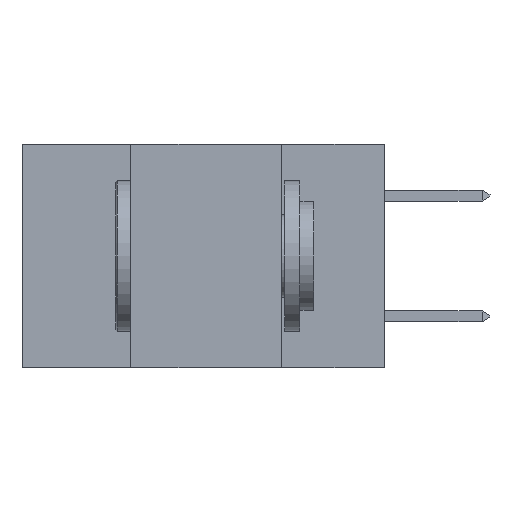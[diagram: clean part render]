
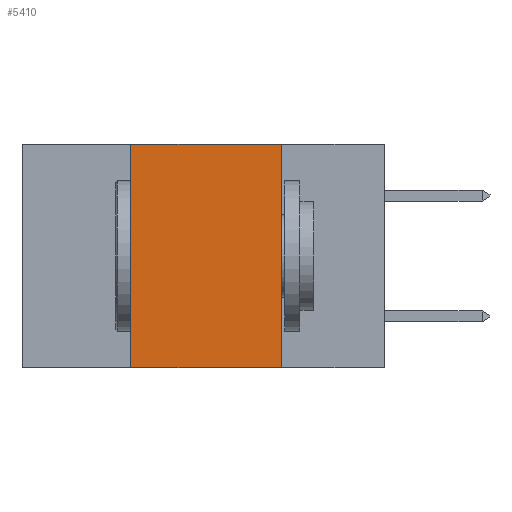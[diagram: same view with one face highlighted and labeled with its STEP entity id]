
A CAD part, left-side view. The second image highlights one B-rep face of the part: STEP entity #5410.
In plain terms, the highlighted planar face has unit normal (-1, 0, 0).
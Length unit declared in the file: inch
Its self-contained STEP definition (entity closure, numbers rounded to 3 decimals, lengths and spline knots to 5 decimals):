
#563 = VECTOR ( 'NONE', #12512, 39.37008 ) ;
#585 = LINE ( 'NONE', #1624, #803 ) ;
#803 = VECTOR ( 'NONE', #5555, 39.37008 ) ;
#886 = ORIENTED_EDGE ( 'NONE', *, *, #1706, .F. ) ;
#1472 = DIRECTION ( 'NONE',  ( 1., 0., 0. ) ) ;
#1624 = CARTESIAN_POINT ( 'NONE',  ( 0., 0.42, 0. ) ) ;
#1706 = EDGE_CURVE ( 'NONE', #14833, #10369, #585, .T. ) ;
#1783 = FACE_OUTER_BOUND ( 'NONE', #3648, .T. ) ;
#2396 = CARTESIAN_POINT ( 'NONE',  ( 0., 0.6, 0. ) ) ;
#2452 = EDGE_CURVE ( 'NONE', #4862, #13947, #6821, .T. ) ;
#3122 = CARTESIAN_POINT ( 'NONE',  ( 0., 0.17, 0. ) ) ;
#3648 = EDGE_LOOP ( 'NONE', ( #11892, #12682, #886, #4486 ) ) ;
#3963 = PLANE ( 'NONE',  #13279 ) ;
#4116 = CARTESIAN_POINT ( 'NONE',  ( 0., 0.42, 0. ) ) ;
#4486 = ORIENTED_EDGE ( 'NONE', *, *, #10603, .T. ) ;
#4862 = VERTEX_POINT ( 'NONE', #6305 ) ;
#5409 = VECTOR ( 'NONE', #9842, 39.37008 ) ;
#5410 = ADVANCED_FACE ( 'NONE', ( #1783 ), #3963, .F. ) ;
#5555 = DIRECTION ( 'NONE',  ( 0., 0., 1. ) ) ;
#6305 = CARTESIAN_POINT ( 'NONE',  ( 0., 0.17, 0. ) ) ;
#6821 = LINE ( 'NONE', #3122, #5409 ) ;
#7088 = LINE ( 'NONE', #2396, #16098 ) ;
#7910 = CARTESIAN_POINT ( 'NONE',  ( 0., 0.17, -0.37 ) ) ;
#8180 = CARTESIAN_POINT ( 'NONE',  ( 0., 0.42, -0.37 ) ) ;
#9359 = CARTESIAN_POINT ( 'NONE',  ( 0., 0.6, 0. ) ) ;
#9842 = DIRECTION ( 'NONE',  ( 0., 0., -1. ) ) ;
#10369 = VERTEX_POINT ( 'NONE', #4116 ) ;
#10497 = DIRECTION ( 'NONE',  ( 0., 0., -1. ) ) ;
#10603 = EDGE_CURVE ( 'NONE', #14833, #13947, #15557, .T. ) ;
#11892 = ORIENTED_EDGE ( 'NONE', *, *, #2452, .F. ) ;
#12512 = DIRECTION ( 'NONE',  ( 0., -1., 0. ) ) ;
#12664 = EDGE_CURVE ( 'NONE', #10369, #4862, #7088, .T. ) ;
#12682 = ORIENTED_EDGE ( 'NONE', *, *, #12664, .F. ) ;
#13279 = AXIS2_PLACEMENT_3D ( 'NONE', #9359, #1472, #10497 ) ;
#13561 = CARTESIAN_POINT ( 'NONE',  ( 0., 0.6, -0.37 ) ) ;
#13947 = VERTEX_POINT ( 'NONE', #7910 ) ;
#13970 = DIRECTION ( 'NONE',  ( 0., -1., 0. ) ) ;
#14833 = VERTEX_POINT ( 'NONE', #8180 ) ;
#15557 = LINE ( 'NONE', #13561, #563 ) ;
#16098 = VECTOR ( 'NONE', #13970, 39.37008 ) ;
